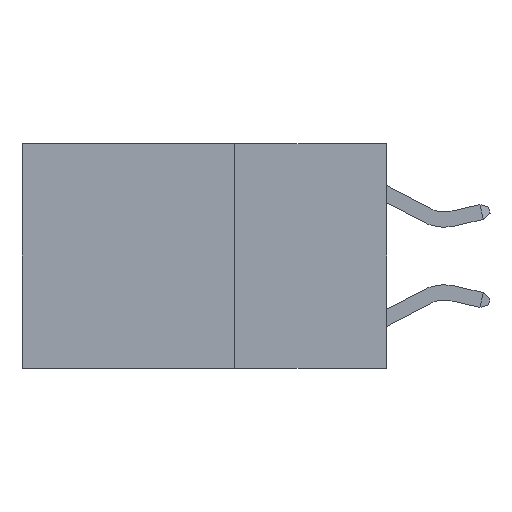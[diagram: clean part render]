
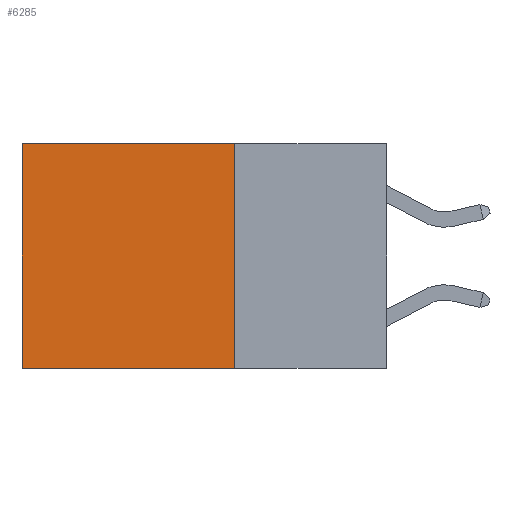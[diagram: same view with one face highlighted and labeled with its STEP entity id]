
A CAD part, left-side view. The second image highlights one B-rep face of the part: STEP entity #6285.
In plain terms, the highlighted planar face has unit normal (-1, 0, 0).
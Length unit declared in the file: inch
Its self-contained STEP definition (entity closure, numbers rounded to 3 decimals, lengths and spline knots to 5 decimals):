
#113 = VERTEX_POINT ( 'NONE', #2279 ) ;
#1187 = ORIENTED_EDGE ( 'NONE', *, *, #13742, .T. ) ;
#2279 = CARTESIAN_POINT ( 'NONE',  ( 0.2625, 0.6, -0.37 ) ) ;
#3145 = ORIENTED_EDGE ( 'NONE', *, *, #5694, .T. ) ;
#3686 = CARTESIAN_POINT ( 'NONE',  ( 0.2625, 0.25, 0. ) ) ;
#4041 = DIRECTION ( 'NONE',  ( 0., 1., 0. ) ) ;
#4469 = VECTOR ( 'NONE', #23144, 39.37008 ) ;
#5625 = DIRECTION ( 'NONE',  ( 0., 0., -1. ) ) ;
#5694 = EDGE_CURVE ( 'NONE', #9094, #113, #10203, .T. ) ;
#5906 = CARTESIAN_POINT ( 'NONE',  ( 0.2625, 0.25, 0. ) ) ;
#6285 = ADVANCED_FACE ( 'NONE', ( #11592 ), #16746, .F. ) ;
#6690 = ORIENTED_EDGE ( 'NONE', *, *, #7804, .F. ) ;
#7050 = CARTESIAN_POINT ( 'NONE',  ( 0.2625, 0.6, 0. ) ) ;
#7487 = AXIS2_PLACEMENT_3D ( 'NONE', #3686, #11246, #24163 ) ;
#7804 = EDGE_CURVE ( 'NONE', #21836, #113, #15004, .T. ) ;
#8431 = VECTOR ( 'NONE', #19124, 39.37008 ) ;
#8737 = EDGE_LOOP ( 'NONE', ( #3145, #6690, #18577, #1187 ) ) ;
#9094 = VERTEX_POINT ( 'NONE', #7050 ) ;
#9350 = CARTESIAN_POINT ( 'NONE',  ( 0.2625, 0.6, 0. ) ) ;
#10203 = LINE ( 'NONE', #9350, #18906 ) ;
#10546 = EDGE_CURVE ( 'NONE', #22036, #21836, #18307, .T. ) ;
#11246 = DIRECTION ( 'NONE',  ( 1., 0., 0. ) ) ;
#11592 = FACE_OUTER_BOUND ( 'NONE', #8737, .T. ) ;
#12051 = VECTOR ( 'NONE', #4041, 39.37008 ) ;
#13742 = EDGE_CURVE ( 'NONE', #22036, #9094, #20776, .T. ) ;
#15004 = LINE ( 'NONE', #17680, #4469 ) ;
#15222 = CARTESIAN_POINT ( 'NONE',  ( 0.2625, 0.25, 0. ) ) ;
#15356 = CARTESIAN_POINT ( 'NONE',  ( 0.2625, 0.25, 0. ) ) ;
#16746 = PLANE ( 'NONE',  #7487 ) ;
#17680 = CARTESIAN_POINT ( 'NONE',  ( 0.2625, 0.25, -0.37 ) ) ;
#18307 = LINE ( 'NONE', #15356, #8431 ) ;
#18577 = ORIENTED_EDGE ( 'NONE', *, *, #10546, .F. ) ;
#18906 = VECTOR ( 'NONE', #5625, 39.37008 ) ;
#19124 = DIRECTION ( 'NONE',  ( 0., 0., -1. ) ) ;
#20776 = LINE ( 'NONE', #15222, #12051 ) ;
#21836 = VERTEX_POINT ( 'NONE', #23915 ) ;
#22036 = VERTEX_POINT ( 'NONE', #5906 ) ;
#23144 = DIRECTION ( 'NONE',  ( 0., 1., 0. ) ) ;
#23915 = CARTESIAN_POINT ( 'NONE',  ( 0.2625, 0.25, -0.37 ) ) ;
#24163 = DIRECTION ( 'NONE',  ( 0., 0., -1. ) ) ;
